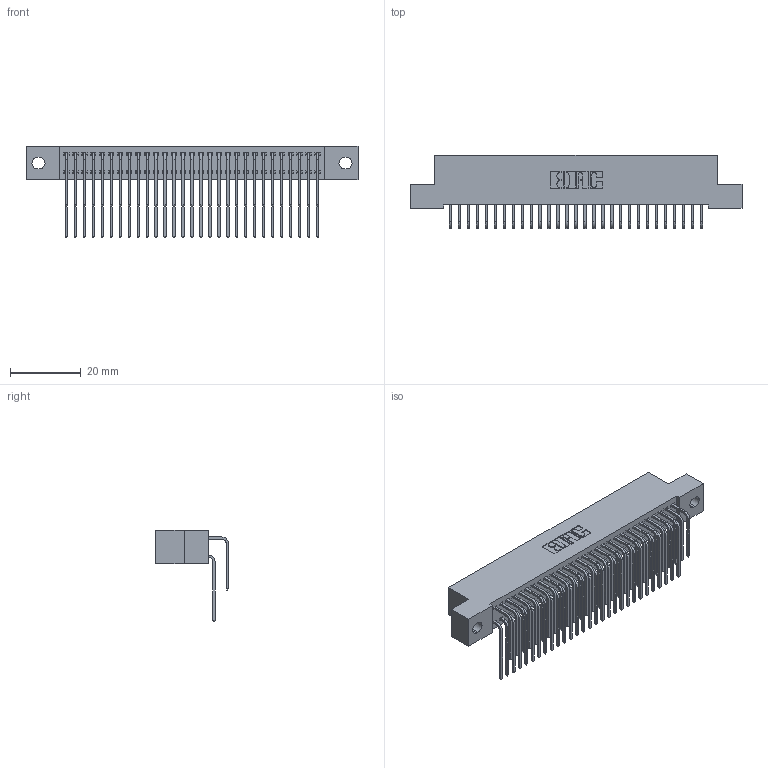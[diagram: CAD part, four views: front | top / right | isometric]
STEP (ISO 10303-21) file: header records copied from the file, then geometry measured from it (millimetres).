
FILE_DESCRIPTION (( 'STEP AP203' ), '1' );
FILE_NAME ('392-058-559-202.STEP', '2018-08-17T18:29:53', ( '' ), ( '' ), 'SwSTEP 2.0', 'SolidWorks 2016', '' );
FILE_SCHEMA (( 'CONFIG_CONTROL_DESIGN' ));
Length unit declared in the file: inch
Products named in the file (4): 342 Part_.128 Slot; 345-292-001_558 559 Tail - 1; 345-292-001_559 Tail - 2; 392-058-559-202
Assembly tree (59 placements, depth 2):
  392-058-559-202
    342 Part_.128 Slot
    345-292-001_558 559 Tail - 1  x29
    345-292-001_559 Tail - 2  x29
Bounding box: 93.98 x 20.64 x 25.78 mm (x, y, z)
Volume: 8665 mm3; surface area: 15057.2 mm2
Topology: 59 solids, 59 shells, 3246 faces, 9649 edges, 6354 vertices
Faces by surface type: plane 2274, cylinder 972
Entity records: 22125 total; most frequent: CARTESIAN_POINT 3733, ORIENTED_EDGE 3618, DIRECTION 3193, EDGE_CURVE 1809, VECTOR 1641, LINE 1641, VERTEX_POINT 1202, AXIS2_PLACEMENT_3D 776
